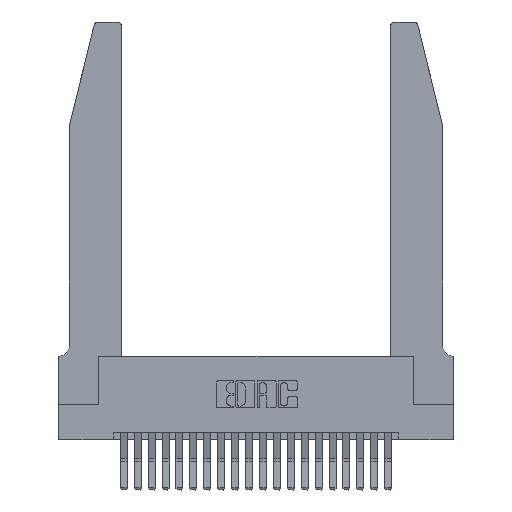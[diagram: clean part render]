
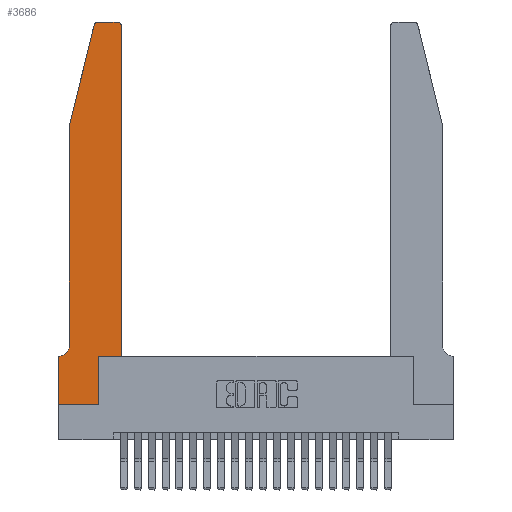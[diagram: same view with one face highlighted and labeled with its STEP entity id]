
A CAD part, top view. The second image highlights one B-rep face of the part: STEP entity #3686.
In plain terms, the highlighted planar face has unit normal (0, 0, 1).
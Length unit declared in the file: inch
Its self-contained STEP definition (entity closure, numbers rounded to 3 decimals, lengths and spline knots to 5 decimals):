
#262 = CARTESIAN_POINT ( 'NONE',  ( 0.4205, 2.72, 0.37 ) ) ;
#984 = FACE_OUTER_BOUND ( 'NONE', #17217, .T. ) ;
#986 = VERTEX_POINT ( 'NONE', #12338 ) ;
#1259 = LINE ( 'NONE', #6553, #11158 ) ;
#1619 = EDGE_CURVE ( 'NONE', #5863, #20312, #11213, .T. ) ;
#1724 = DIRECTION ( 'NONE',  ( 0., -1., 0. ) ) ;
#1795 = CARTESIAN_POINT ( 'NONE',  ( 0., 0., 0.37 ) ) ;
#2007 = AXIS2_PLACEMENT_3D ( 'NONE', #7576, #15005, #20226 ) ;
#2235 = CARTESIAN_POINT ( 'NONE',  ( 0., 0.35, 0.37 ) ) ;
#2418 = VERTEX_POINT ( 'NONE', #18209 ) ;
#2428 = EDGE_CURVE ( 'NONE', #3025, #10693, #5818, .T. ) ;
#2682 = VERTEX_POINT ( 'NONE', #6102 ) ;
#2922 = DIRECTION ( 'NONE',  ( 0., 0., -1. ) ) ;
#3025 = VERTEX_POINT ( 'NONE', #21710 ) ;
#3146 = CARTESIAN_POINT ( 'NONE',  ( 0.2865, 0., 0.37 ) ) ;
#3323 = DIRECTION ( 'NONE',  ( 1., 0., 0. ) ) ;
#3686 = ADVANCED_FACE ( 'NONE', ( #984 ), #23257, .T. ) ;
#3923 = VERTEX_POINT ( 'NONE', #9850 ) ;
#4403 = VECTOR ( 'NONE', #1724, 39.37008 ) ;
#4463 = ORIENTED_EDGE ( 'NONE', *, *, #22337, .T. ) ;
#4469 = DIRECTION ( 'NONE',  ( -1., 0., 0. ) ) ;
#4569 = LINE ( 'NONE', #20054, #21942 ) ;
#4992 = VECTOR ( 'NONE', #23522, 39.37008 ) ;
#5062 = EDGE_CURVE ( 'NONE', #20312, #5354, #4569, .T. ) ;
#5342 = VECTOR ( 'NONE', #14647, 39.37008 ) ;
#5354 = VERTEX_POINT ( 'NONE', #10530 ) ;
#5545 = VECTOR ( 'NONE', #16364, 39.37008 ) ;
#5818 = LINE ( 'NONE', #22115, #5545 ) ;
#5863 = VERTEX_POINT ( 'NONE', #1795 ) ;
#6007 = CARTESIAN_POINT ( 'NONE',  ( 0.0755, 0.35, 0.37 ) ) ;
#6102 = CARTESIAN_POINT ( 'NONE',  ( 0.4505, 0.35, 0.37 ) ) ;
#6114 = CARTESIAN_POINT ( 'NONE',  ( 0.4505, 0.35, 0.37 ) ) ;
#6512 = ORIENTED_EDGE ( 'NONE', *, *, #9845, .T. ) ;
#6553 = CARTESIAN_POINT ( 'NONE',  ( 0.2605, 2.75, 0.37 ) ) ;
#7139 = CARTESIAN_POINT ( 'NONE',  ( 0., 0., 0.37 ) ) ;
#7331 = CIRCLE ( 'NONE', #2007, 0.03 ) ;
#7576 = CARTESIAN_POINT ( 'NONE',  ( 0.284, 2.72, 0.37 ) ) ;
#7744 = EDGE_CURVE ( 'NONE', #22213, #3923, #1259, .T. ) ;
#8900 = ORIENTED_EDGE ( 'NONE', *, *, #12989, .T. ) ;
#8957 = CARTESIAN_POINT ( 'NONE',  ( 0.4205, 2.75, 0.37 ) ) ;
#8996 = ORIENTED_EDGE ( 'NONE', *, *, #7744, .T. ) ;
#9054 = VERTEX_POINT ( 'NONE', #2235 ) ;
#9059 = VECTOR ( 'NONE', #14779, 39.37008 ) ;
#9425 = LINE ( 'NONE', #11173, #21987 ) ;
#9599 = ORIENTED_EDGE ( 'NONE', *, *, #18325, .T. ) ;
#9845 = EDGE_CURVE ( 'NONE', #2418, #3025, #14124, .T. ) ;
#9850 = CARTESIAN_POINT ( 'NONE',  ( 0.284, 2.75, 0.37 ) ) ;
#10530 = CARTESIAN_POINT ( 'NONE',  ( 0.2865, 0.35, 0.37 ) ) ;
#10693 = VERTEX_POINT ( 'NONE', #18895 ) ;
#11158 = VECTOR ( 'NONE', #19427, 39.37008 ) ;
#11173 = CARTESIAN_POINT ( 'NONE',  ( 0.4505, 0.35, 0.37 ) ) ;
#11213 = LINE ( 'NONE', #7139, #4992 ) ;
#11300 = LINE ( 'NONE', #6007, #9059 ) ;
#11395 = ORIENTED_EDGE ( 'NONE', *, *, #14603, .T. ) ;
#11662 = DIRECTION ( 'NONE',  ( 1., 0., 0. ) ) ;
#12338 = CARTESIAN_POINT ( 'NONE',  ( 0.4505, 2.72, 0.37 ) ) ;
#12782 = AXIS2_PLACEMENT_3D ( 'NONE', #262, #22754, #11662 ) ;
#12959 = EDGE_CURVE ( 'NONE', #5354, #2682, #9425, .T. ) ;
#12969 = CARTESIAN_POINT ( 'NONE',  ( 0.0755, 2., 0.37 ) ) ;
#12989 = EDGE_CURVE ( 'NONE', #2682, #986, #22557, .T. ) ;
#13000 = ORIENTED_EDGE ( 'NONE', *, *, #15673, .T. ) ;
#13269 = AXIS2_PLACEMENT_3D ( 'NONE', #13755, #2922, #4469 ) ;
#13672 = VECTOR ( 'NONE', #18606, 39.37008 ) ;
#13755 = CARTESIAN_POINT ( 'NONE',  ( 0.0055, 0.42, 0.37 ) ) ;
#14124 = LINE ( 'NONE', #12969, #5342 ) ;
#14603 = EDGE_CURVE ( 'NONE', #9054, #5863, #20894, .T. ) ;
#14647 = DIRECTION ( 'NONE',  ( -0.239, -0.971, 0. ) ) ;
#14779 = DIRECTION ( 'NONE',  ( -1., 0., 0. ) ) ;
#14957 = EDGE_CURVE ( 'NONE', #3923, #2418, #7331, .T. ) ;
#15005 = DIRECTION ( 'NONE',  ( 0., 0., 1. ) ) ;
#15056 = DIRECTION ( 'NONE',  ( 1., 0., 0. ) ) ;
#15299 = ORIENTED_EDGE ( 'NONE', *, *, #1619, .T. ) ;
#15673 = EDGE_CURVE ( 'NONE', #986, #22213, #21535, .T. ) ;
#16358 = CARTESIAN_POINT ( 'NONE',  ( 0.0055, 0.35, 0.37 ) ) ;
#16364 = DIRECTION ( 'NONE',  ( 0., -1., 0. ) ) ;
#16453 = DIRECTION ( 'NONE',  ( 0., 1., 0. ) ) ;
#16937 = ORIENTED_EDGE ( 'NONE', *, *, #5062, .T. ) ;
#17217 = EDGE_LOOP ( 'NONE', ( #8996, #22309, #6512, #18440, #9599, #4463, #11395, #15299, #16937, #22988, #8900, #13000 ) ) ;
#17845 = DIRECTION ( 'NONE',  ( 0., 0., 1. ) ) ;
#18209 = CARTESIAN_POINT ( 'NONE',  ( 0.25487, 2.72718, 0.37 ) ) ;
#18325 = EDGE_CURVE ( 'NONE', #10693, #23411, #18534, .T. ) ;
#18440 = ORIENTED_EDGE ( 'NONE', *, *, #2428, .T. ) ;
#18534 = CIRCLE ( 'NONE', #13269, 0.07 ) ;
#18606 = DIRECTION ( 'NONE',  ( 0., 1., 0. ) ) ;
#18895 = CARTESIAN_POINT ( 'NONE',  ( 0.0755, 0.42, 0.37 ) ) ;
#19427 = DIRECTION ( 'NONE',  ( -1., 0., 0. ) ) ;
#19806 = CARTESIAN_POINT ( 'NONE',  ( 0., 0., 0.37 ) ) ;
#20054 = CARTESIAN_POINT ( 'NONE',  ( 0.2865, 0.35, 0.37 ) ) ;
#20226 = DIRECTION ( 'NONE',  ( 1., 0., 0. ) ) ;
#20312 = VERTEX_POINT ( 'NONE', #3146 ) ;
#20894 = LINE ( 'NONE', #19806, #4403 ) ;
#21535 = CIRCLE ( 'NONE', #12782, 0.03 ) ;
#21599 = AXIS2_PLACEMENT_3D ( 'NONE', #23180, #17845, #3323 ) ;
#21710 = CARTESIAN_POINT ( 'NONE',  ( 0.0755, 2., 0.37 ) ) ;
#21942 = VECTOR ( 'NONE', #16453, 39.37008 ) ;
#21987 = VECTOR ( 'NONE', #15056, 39.37008 ) ;
#22115 = CARTESIAN_POINT ( 'NONE',  ( 0.0755, 2., 0.37 ) ) ;
#22213 = VERTEX_POINT ( 'NONE', #8957 ) ;
#22309 = ORIENTED_EDGE ( 'NONE', *, *, #14957, .T. ) ;
#22337 = EDGE_CURVE ( 'NONE', #23411, #9054, #11300, .T. ) ;
#22557 = LINE ( 'NONE', #6114, #13672 ) ;
#22754 = DIRECTION ( 'NONE',  ( 0., 0., 1. ) ) ;
#22988 = ORIENTED_EDGE ( 'NONE', *, *, #12959, .T. ) ;
#23180 = CARTESIAN_POINT ( 'NONE',  ( 0., 0.35, 0.37 ) ) ;
#23257 = PLANE ( 'NONE',  #21599 ) ;
#23411 = VERTEX_POINT ( 'NONE', #16358 ) ;
#23522 = DIRECTION ( 'NONE',  ( 1., 0., 0. ) ) ;
